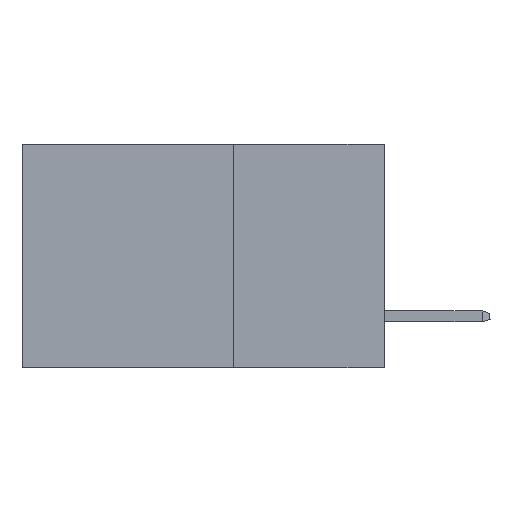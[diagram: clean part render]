
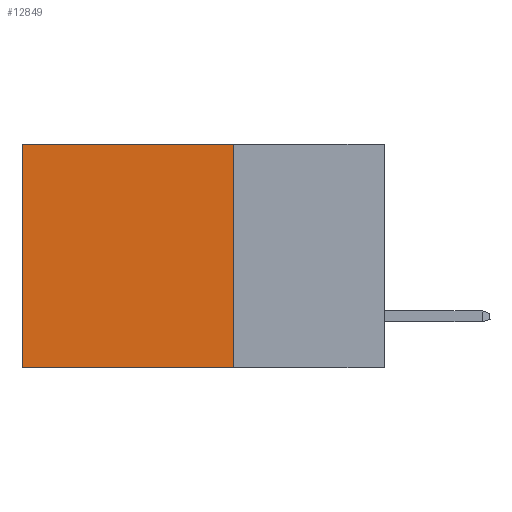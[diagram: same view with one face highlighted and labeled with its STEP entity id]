
A CAD part, left-side view. The second image highlights one B-rep face of the part: STEP entity #12849.
In plain terms, the highlighted planar face has unit normal (-1, 0, 0).
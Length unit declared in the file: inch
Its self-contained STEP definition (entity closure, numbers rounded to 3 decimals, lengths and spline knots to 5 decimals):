
#121 = VECTOR ( 'NONE', #4939, 39.37008 ) ;
#855 = VECTOR ( 'NONE', #2279, 39.37008 ) ;
#1682 = ORIENTED_EDGE ( 'NONE', *, *, #4961, .T. ) ;
#2279 = DIRECTION ( 'NONE',  ( 0., 0., -1. ) ) ;
#2891 = ORIENTED_EDGE ( 'NONE', *, *, #10841, .T. ) ;
#3306 = VECTOR ( 'NONE', #11828, 39.37008 ) ;
#3550 = CARTESIAN_POINT ( 'NONE',  ( 0.298, 0.6, -0.37 ) ) ;
#4769 = CARTESIAN_POINT ( 'NONE',  ( 0.298, 0.25, 0. ) ) ;
#4939 = DIRECTION ( 'NONE',  ( 0., 1., 0. ) ) ;
#4955 = VERTEX_POINT ( 'NONE', #3550 ) ;
#4961 = EDGE_CURVE ( 'NONE', #14880, #5645, #15075, .T. ) ;
#5099 = ORIENTED_EDGE ( 'NONE', *, *, #16520, .F. ) ;
#5287 = LINE ( 'NONE', #16496, #7540 ) ;
#5492 = VERTEX_POINT ( 'NONE', #6164 ) ;
#5605 = PLANE ( 'NONE',  #13187 ) ;
#5645 = VERTEX_POINT ( 'NONE', #12916 ) ;
#5728 = DIRECTION ( 'NONE',  ( 0., 0., -1. ) ) ;
#6164 = CARTESIAN_POINT ( 'NONE',  ( 0.298, 0.25, -0.37 ) ) ;
#6205 = LINE ( 'NONE', #10557, #3306 ) ;
#6978 = DIRECTION ( 'NONE',  ( 1., 0., 0. ) ) ;
#7540 = VECTOR ( 'NONE', #16662, 39.37008 ) ;
#8298 = LINE ( 'NONE', #14010, #855 ) ;
#10557 = CARTESIAN_POINT ( 'NONE',  ( 0.298, 0.25, -0.37 ) ) ;
#10841 = EDGE_CURVE ( 'NONE', #5645, #4955, #5287, .T. ) ;
#11828 = DIRECTION ( 'NONE',  ( 0., 1., 0. ) ) ;
#12847 = CARTESIAN_POINT ( 'NONE',  ( 0.298, 0.25, 0. ) ) ;
#12849 = ADVANCED_FACE ( 'NONE', ( #14077 ), #5605, .F. ) ;
#12916 = CARTESIAN_POINT ( 'NONE',  ( 0.298, 0.6, 0. ) ) ;
#13187 = AXIS2_PLACEMENT_3D ( 'NONE', #14915, #6978, #5728 ) ;
#14010 = CARTESIAN_POINT ( 'NONE',  ( 0.298, 0.25, 0. ) ) ;
#14077 = FACE_OUTER_BOUND ( 'NONE', #15827, .T. ) ;
#14880 = VERTEX_POINT ( 'NONE', #12847 ) ;
#14915 = CARTESIAN_POINT ( 'NONE',  ( 0.298, 0.25, 0. ) ) ;
#15075 = LINE ( 'NONE', #4769, #121 ) ;
#15827 = EDGE_LOOP ( 'NONE', ( #2891, #16436, #5099, #1682 ) ) ;
#16436 = ORIENTED_EDGE ( 'NONE', *, *, #16715, .F. ) ;
#16496 = CARTESIAN_POINT ( 'NONE',  ( 0.298, 0.6, 0. ) ) ;
#16520 = EDGE_CURVE ( 'NONE', #14880, #5492, #8298, .T. ) ;
#16662 = DIRECTION ( 'NONE',  ( 0., 0., -1. ) ) ;
#16715 = EDGE_CURVE ( 'NONE', #5492, #4955, #6205, .T. ) ;
